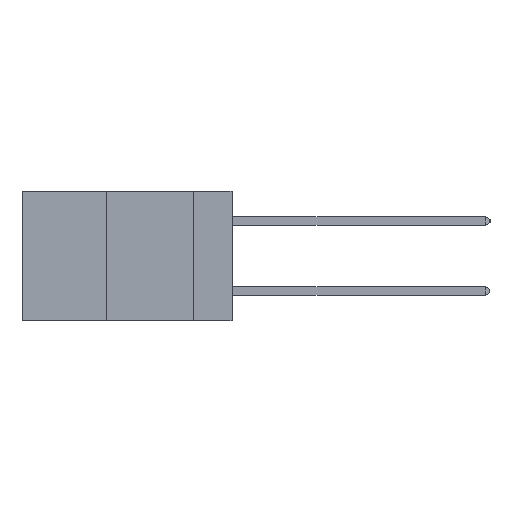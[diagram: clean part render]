
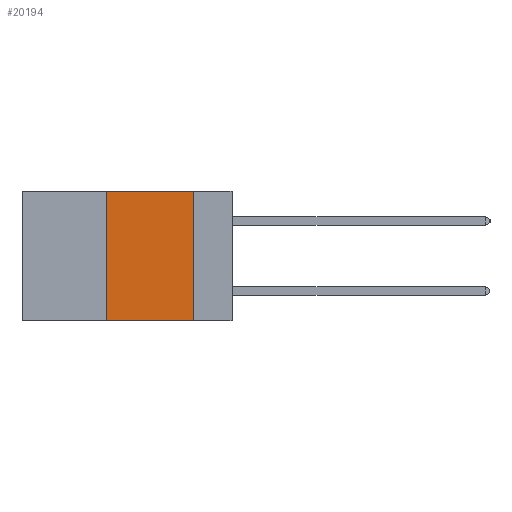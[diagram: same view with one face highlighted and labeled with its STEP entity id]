
A CAD part, left-side view. The second image highlights one B-rep face of the part: STEP entity #20194.
In plain terms, the highlighted planar face has unit normal (-1, 0, 0).
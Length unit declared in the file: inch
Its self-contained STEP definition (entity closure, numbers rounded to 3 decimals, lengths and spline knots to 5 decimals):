
#1007 = DIRECTION ( 'NONE',  ( 0., -1., 0. ) ) ;
#1373 = LINE ( 'NONE', #21285, #10689 ) ;
#1481 = ORIENTED_EDGE ( 'NONE', *, *, #6179, .F. ) ;
#1987 = VERTEX_POINT ( 'NONE', #20809 ) ;
#2295 = PLANE ( 'NONE',  #3638 ) ;
#2615 = LINE ( 'NONE', #11493, #17114 ) ;
#2825 = LINE ( 'NONE', #11110, #12098 ) ;
#3638 = AXIS2_PLACEMENT_3D ( 'NONE', #14529, #4036, #16311 ) ;
#4036 = DIRECTION ( 'NONE',  ( 1., 0., 0. ) ) ;
#4454 = FACE_OUTER_BOUND ( 'NONE', #19953, .T. ) ;
#4968 = EDGE_CURVE ( 'NONE', #7702, #10451, #2825, .T. ) ;
#5267 = ORIENTED_EDGE ( 'NONE', *, *, #21747, .T. ) ;
#5489 = VECTOR ( 'NONE', #6932, 39.37008 ) ;
#6062 = LINE ( 'NONE', #20785, #5489 ) ;
#6179 = EDGE_CURVE ( 'NONE', #7241, #1987, #1373, .T. ) ;
#6932 = DIRECTION ( 'NONE',  ( 0., -1., 0. ) ) ;
#7071 = ORIENTED_EDGE ( 'NONE', *, *, #13437, .F. ) ;
#7241 = VERTEX_POINT ( 'NONE', #20646 ) ;
#7638 = ORIENTED_EDGE ( 'NONE', *, *, #4968, .F. ) ;
#7702 = VERTEX_POINT ( 'NONE', #13204 ) ;
#8474 = DIRECTION ( 'NONE',  ( 0., 0., -1. ) ) ;
#9096 = DIRECTION ( 'NONE',  ( 0., 0., 1. ) ) ;
#10451 = VERTEX_POINT ( 'NONE', #21167 ) ;
#10689 = VECTOR ( 'NONE', #9096, 39.37008 ) ;
#11110 = CARTESIAN_POINT ( 'NONE',  ( 0., 0.11, 0. ) ) ;
#11493 = CARTESIAN_POINT ( 'NONE',  ( 0., 0.6, -0.37 ) ) ;
#12098 = VECTOR ( 'NONE', #8474, 39.37008 ) ;
#13204 = CARTESIAN_POINT ( 'NONE',  ( 0., 0.11, 0. ) ) ;
#13437 = EDGE_CURVE ( 'NONE', #1987, #7702, #6062, .T. ) ;
#14529 = CARTESIAN_POINT ( 'NONE',  ( 0., 0.6, 0. ) ) ;
#16311 = DIRECTION ( 'NONE',  ( 0., 0., -1. ) ) ;
#17114 = VECTOR ( 'NONE', #1007, 39.37008 ) ;
#19953 = EDGE_LOOP ( 'NONE', ( #7638, #7071, #1481, #5267 ) ) ;
#20194 = ADVANCED_FACE ( 'NONE', ( #4454 ), #2295, .F. ) ;
#20646 = CARTESIAN_POINT ( 'NONE',  ( 0., 0.36, -0.37 ) ) ;
#20785 = CARTESIAN_POINT ( 'NONE',  ( 0., 0.6, 0. ) ) ;
#20809 = CARTESIAN_POINT ( 'NONE',  ( 0., 0.36, 0. ) ) ;
#21167 = CARTESIAN_POINT ( 'NONE',  ( 0., 0.11, -0.37 ) ) ;
#21285 = CARTESIAN_POINT ( 'NONE',  ( 0., 0.36, 0. ) ) ;
#21747 = EDGE_CURVE ( 'NONE', #7241, #10451, #2615, .T. ) ;
